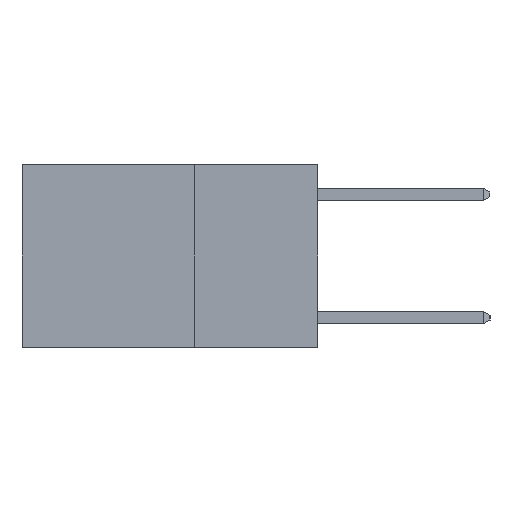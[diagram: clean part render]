
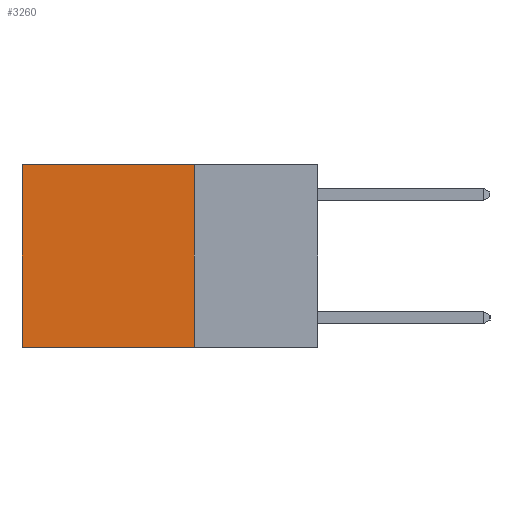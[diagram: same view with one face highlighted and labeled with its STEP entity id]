
A CAD part, left-side view. The second image highlights one B-rep face of the part: STEP entity #3260.
In plain terms, the highlighted planar face has unit normal (-1, 0, 0).
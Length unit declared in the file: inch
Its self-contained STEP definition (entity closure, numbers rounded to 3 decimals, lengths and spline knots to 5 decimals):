
#169 = CARTESIAN_POINT ( 'NONE',  ( 0.2625, 0.6, -0.37 ) ) ;
#212 = ORIENTED_EDGE ( 'NONE', *, *, #2380, .F. ) ;
#736 = DIRECTION ( 'NONE',  ( 0., 1., 0. ) ) ;
#765 = VERTEX_POINT ( 'NONE', #169 ) ;
#800 = CARTESIAN_POINT ( 'NONE',  ( 0.2625, 0.25, 0. ) ) ;
#903 = EDGE_LOOP ( 'NONE', ( #8353, #2750, #212, #4930 ) ) ;
#1111 = EDGE_CURVE ( 'NONE', #1916, #765, #3025, .T. ) ;
#1125 = VERTEX_POINT ( 'NONE', #5156 ) ;
#1408 = AXIS2_PLACEMENT_3D ( 'NONE', #3498, #8643, #4974 ) ;
#1449 = EDGE_CURVE ( 'NONE', #1125, #765, #8331, .T. ) ;
#1916 = VERTEX_POINT ( 'NONE', #5557 ) ;
#2380 = EDGE_CURVE ( 'NONE', #6646, #1125, #2452, .T. ) ;
#2452 = LINE ( 'NONE', #5348, #8124 ) ;
#2750 = ORIENTED_EDGE ( 'NONE', *, *, #1449, .F. ) ;
#3025 = LINE ( 'NONE', #9693, #6722 ) ;
#3260 = ADVANCED_FACE ( 'NONE', ( #3959 ), #4233, .F. ) ;
#3376 = CARTESIAN_POINT ( 'NONE',  ( 0.2625, 0.25, 0. ) ) ;
#3498 = CARTESIAN_POINT ( 'NONE',  ( 0.2625, 0.25, 0. ) ) ;
#3959 = FACE_OUTER_BOUND ( 'NONE', #903, .T. ) ;
#4233 = PLANE ( 'NONE',  #1408 ) ;
#4513 = DIRECTION ( 'NONE',  ( 0., 0., -1. ) ) ;
#4930 = ORIENTED_EDGE ( 'NONE', *, *, #9050, .T. ) ;
#4974 = DIRECTION ( 'NONE',  ( 0., 0., -1. ) ) ;
#5156 = CARTESIAN_POINT ( 'NONE',  ( 0.2625, 0.25, -0.37 ) ) ;
#5348 = CARTESIAN_POINT ( 'NONE',  ( 0.2625, 0.25, 0. ) ) ;
#5531 = VECTOR ( 'NONE', #8535, 39.37008 ) ;
#5557 = CARTESIAN_POINT ( 'NONE',  ( 0.2625, 0.6, 0. ) ) ;
#6161 = VECTOR ( 'NONE', #736, 39.37008 ) ;
#6646 = VERTEX_POINT ( 'NONE', #800 ) ;
#6722 = VECTOR ( 'NONE', #4513, 39.37008 ) ;
#7877 = CARTESIAN_POINT ( 'NONE',  ( 0.2625, 0.25, -0.37 ) ) ;
#8124 = VECTOR ( 'NONE', #9057, 39.37008 ) ;
#8331 = LINE ( 'NONE', #7877, #6161 ) ;
#8353 = ORIENTED_EDGE ( 'NONE', *, *, #1111, .T. ) ;
#8535 = DIRECTION ( 'NONE',  ( 0., 1., 0. ) ) ;
#8643 = DIRECTION ( 'NONE',  ( 1., 0., 0. ) ) ;
#9050 = EDGE_CURVE ( 'NONE', #6646, #1916, #9258, .T. ) ;
#9057 = DIRECTION ( 'NONE',  ( 0., 0., -1. ) ) ;
#9258 = LINE ( 'NONE', #3376, #5531 ) ;
#9693 = CARTESIAN_POINT ( 'NONE',  ( 0.2625, 0.6, 0. ) ) ;
